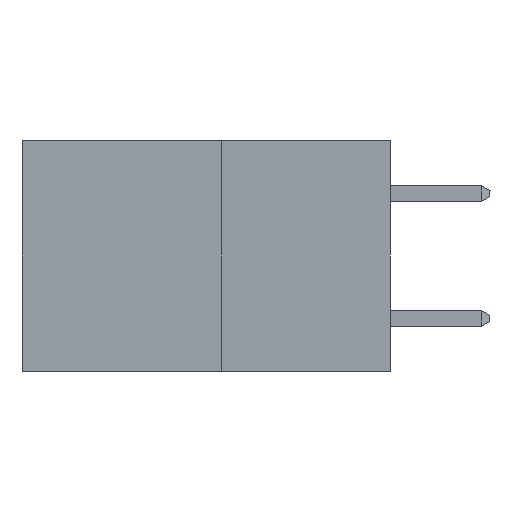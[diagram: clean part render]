
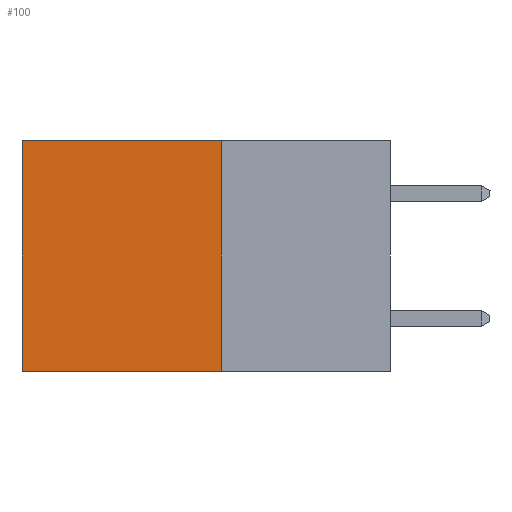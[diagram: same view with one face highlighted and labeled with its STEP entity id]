
A CAD part, left-side view. The second image highlights one B-rep face of the part: STEP entity #100.
In plain terms, the highlighted planar face has unit normal (-1, 0, 0).
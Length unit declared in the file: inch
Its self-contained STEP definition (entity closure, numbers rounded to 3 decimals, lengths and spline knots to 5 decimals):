
#100 = ADVANCED_FACE ( 'NONE', ( #4627 ), #5821, .F. ) ;
#124 = CARTESIAN_POINT ( 'NONE',  ( 0.277, 0.59, -0.37 ) ) ;
#125 = ORIENTED_EDGE ( 'NONE', *, *, #7897, .T. ) ;
#211 = CARTESIAN_POINT ( 'NONE',  ( 0.277, 0.27, -0.37 ) ) ;
#252 = DIRECTION ( 'NONE',  ( 0., 1., 0. ) ) ;
#299 = ORIENTED_EDGE ( 'NONE', *, *, #7346, .F. ) ;
#721 = LINE ( 'NONE', #124, #6127 ) ;
#823 = ORIENTED_EDGE ( 'NONE', *, *, #1475, .F. ) ;
#942 = VERTEX_POINT ( 'NONE', #2903 ) ;
#1119 = CARTESIAN_POINT ( 'NONE',  ( 0.277, 0.27, -0.37 ) ) ;
#1446 = VERTEX_POINT ( 'NONE', #1119 ) ;
#1475 = EDGE_CURVE ( 'NONE', #1716, #1446, #5865, .T. ) ;
#1716 = VERTEX_POINT ( 'NONE', #6886 ) ;
#2061 = ORIENTED_EDGE ( 'NONE', *, *, #7733, .T. ) ;
#2903 = CARTESIAN_POINT ( 'NONE',  ( 0.277, 0.59, 0. ) ) ;
#3904 = LINE ( 'NONE', #6942, #7035 ) ;
#4627 = FACE_OUTER_BOUND ( 'NONE', #4776, .T. ) ;
#4776 = EDGE_LOOP ( 'NONE', ( #2061, #299, #823, #125 ) ) ;
#4853 = CARTESIAN_POINT ( 'NONE',  ( 0.277, 0.59, -0.37 ) ) ;
#5821 = PLANE ( 'NONE',  #6596 ) ;
#5858 = DIRECTION ( 'NONE',  ( 0., 0., -1. ) ) ;
#5865 = LINE ( 'NONE', #211, #7362 ) ;
#5934 = DIRECTION ( 'NONE',  ( 0., 0., -1. ) ) ;
#6105 = CARTESIAN_POINT ( 'NONE',  ( 0.277, 0.27, -0.37 ) ) ;
#6127 = VECTOR ( 'NONE', #5858, 39.37008 ) ;
#6130 = DIRECTION ( 'NONE',  ( 1., 0., 0. ) ) ;
#6596 = AXIS2_PLACEMENT_3D ( 'NONE', #6105, #6130, #5934 ) ;
#6630 = CARTESIAN_POINT ( 'NONE',  ( 0.277, 0.27, 0. ) ) ;
#6639 = VECTOR ( 'NONE', #252, 39.37008 ) ;
#6818 = LINE ( 'NONE', #6630, #6639 ) ;
#6886 = CARTESIAN_POINT ( 'NONE',  ( 0.277, 0.27, 0. ) ) ;
#6942 = CARTESIAN_POINT ( 'NONE',  ( 0.277, 0.27, -0.37 ) ) ;
#7035 = VECTOR ( 'NONE', #7578, 39.37008 ) ;
#7346 = EDGE_CURVE ( 'NONE', #1446, #8143, #3904, .T. ) ;
#7362 = VECTOR ( 'NONE', #8897, 39.37008 ) ;
#7578 = DIRECTION ( 'NONE',  ( 0., 1., 0. ) ) ;
#7733 = EDGE_CURVE ( 'NONE', #942, #8143, #721, .T. ) ;
#7897 = EDGE_CURVE ( 'NONE', #1716, #942, #6818, .T. ) ;
#8143 = VERTEX_POINT ( 'NONE', #4853 ) ;
#8897 = DIRECTION ( 'NONE',  ( 0., 0., -1. ) ) ;
